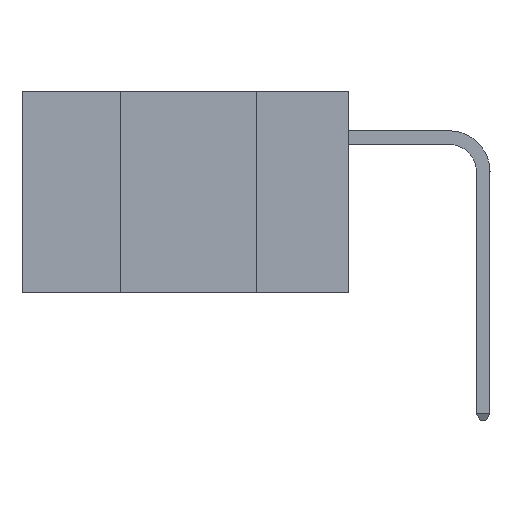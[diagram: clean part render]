
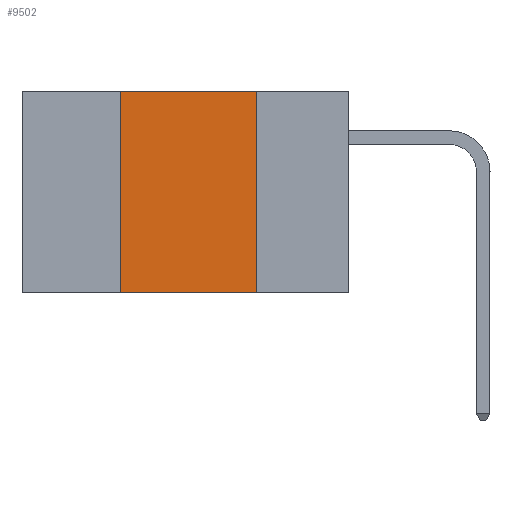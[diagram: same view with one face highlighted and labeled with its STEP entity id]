
A CAD part, left-side view. The second image highlights one B-rep face of the part: STEP entity #9502.
In plain terms, the highlighted planar face has unit normal (-1, 0, 0).
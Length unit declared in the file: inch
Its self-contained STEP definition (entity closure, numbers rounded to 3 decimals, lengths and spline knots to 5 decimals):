
#1422 = CARTESIAN_POINT ( 'NONE',  ( 0., 0.42, -0.37 ) ) ;
#1751 = EDGE_CURVE ( 'NONE', #6889, #10543, #14617, .T. ) ;
#2293 = PLANE ( 'NONE',  #15571 ) ;
#2722 = EDGE_LOOP ( 'NONE', ( #13425, #9390, #8609, #11632 ) ) ;
#3022 = LINE ( 'NONE', #18767, #17083 ) ;
#3125 = LINE ( 'NONE', #12494, #17180 ) ;
#3410 = CARTESIAN_POINT ( 'NONE',  ( 0., 0.42, 0. ) ) ;
#3578 = CARTESIAN_POINT ( 'NONE',  ( 0., 0.42, 0. ) ) ;
#3734 = CARTESIAN_POINT ( 'NONE',  ( 0., 0.17, -0.37 ) ) ;
#3755 = DIRECTION ( 'NONE',  ( 0., 0., -1. ) ) ;
#4692 = EDGE_CURVE ( 'NONE', #9325, #11807, #15416, .T. ) ;
#5342 = DIRECTION ( 'NONE',  ( 0., 0., -1. ) ) ;
#6889 = VERTEX_POINT ( 'NONE', #1422 ) ;
#7720 = VECTOR ( 'NONE', #5342, 39.37008 ) ;
#8609 = ORIENTED_EDGE ( 'NONE', *, *, #1751, .F. ) ;
#8646 = DIRECTION ( 'NONE',  ( 0., -1., 0. ) ) ;
#9325 = VERTEX_POINT ( 'NONE', #14916 ) ;
#9390 = ORIENTED_EDGE ( 'NONE', *, *, #15183, .F. ) ;
#9502 = ADVANCED_FACE ( 'NONE', ( #15105 ), #2293, .F. ) ;
#9658 = CARTESIAN_POINT ( 'NONE',  ( 0., 0.17, 0. ) ) ;
#10543 = VERTEX_POINT ( 'NONE', #3410 ) ;
#11007 = CARTESIAN_POINT ( 'NONE',  ( 0., 0.6, 0. ) ) ;
#11632 = ORIENTED_EDGE ( 'NONE', *, *, #12230, .T. ) ;
#11807 = VERTEX_POINT ( 'NONE', #3734 ) ;
#12056 = DIRECTION ( 'NONE',  ( 0., 0., 1. ) ) ;
#12230 = EDGE_CURVE ( 'NONE', #6889, #11807, #3022, .T. ) ;
#12459 = DIRECTION ( 'NONE',  ( 1., 0., 0. ) ) ;
#12494 = CARTESIAN_POINT ( 'NONE',  ( 0., 0.6, 0. ) ) ;
#13425 = ORIENTED_EDGE ( 'NONE', *, *, #4692, .F. ) ;
#14617 = LINE ( 'NONE', #3578, #17541 ) ;
#14916 = CARTESIAN_POINT ( 'NONE',  ( 0., 0.17, 0. ) ) ;
#15105 = FACE_OUTER_BOUND ( 'NONE', #2722, .T. ) ;
#15183 = EDGE_CURVE ( 'NONE', #10543, #9325, #3125, .T. ) ;
#15416 = LINE ( 'NONE', #9658, #7720 ) ;
#15571 = AXIS2_PLACEMENT_3D ( 'NONE', #11007, #12459, #3755 ) ;
#16816 = DIRECTION ( 'NONE',  ( 0., -1., 0. ) ) ;
#17083 = VECTOR ( 'NONE', #8646, 39.37008 ) ;
#17180 = VECTOR ( 'NONE', #16816, 39.37008 ) ;
#17541 = VECTOR ( 'NONE', #12056, 39.37008 ) ;
#18767 = CARTESIAN_POINT ( 'NONE',  ( 0., 0.6, -0.37 ) ) ;
